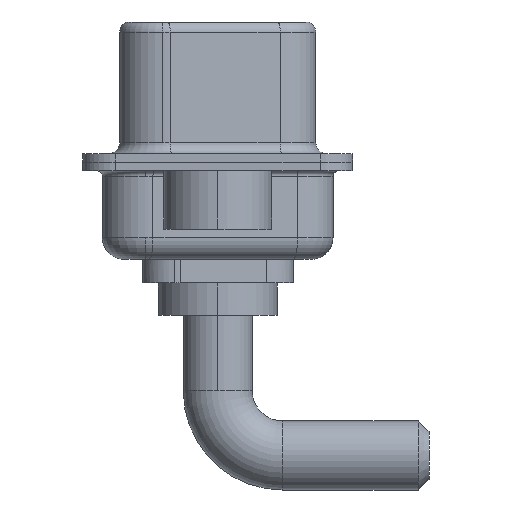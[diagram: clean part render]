
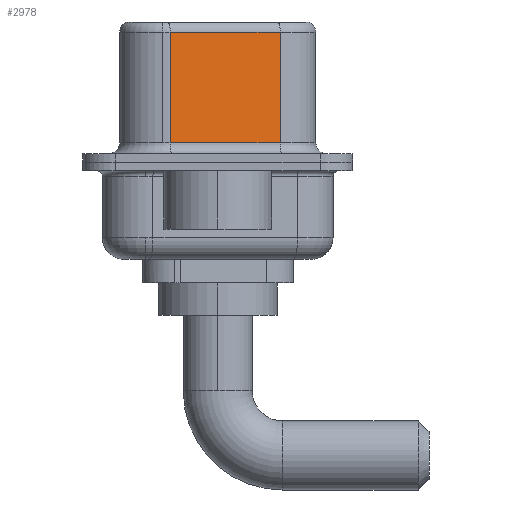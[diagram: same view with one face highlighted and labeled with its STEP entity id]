
A CAD part, left-side view. The second image highlights one B-rep face of the part: STEP entity #2978.
In plain terms, the highlighted planar face has unit normal (-0.985, -0.174, 0).
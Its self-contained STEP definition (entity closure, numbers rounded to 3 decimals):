
#205 = VERTEX_POINT ( 'NONE', #13183 ) ;
#324 = DIRECTION ( 'NONE',  ( 0.174, -0.985, 0. ) ) ;
#850 = ORIENTED_EDGE ( 'NONE', *, *, #14036, .T. ) ;
#1481 = LINE ( 'NONE', #4969, #8563 ) ;
#1835 = ORIENTED_EDGE ( 'NONE', *, *, #7046, .F. ) ;
#1905 = CARTESIAN_POINT ( 'NONE',  ( 4.58, -2.897, 6.52 ) ) ;
#2580 = DIRECTION ( 'NONE',  ( -0.174, 0.985, 0. ) ) ;
#2842 = CARTESIAN_POINT ( 'NONE',  ( 4.58, -2.897, 6.02 ) ) ;
#2854 = LINE ( 'NONE', #1905, #4790 ) ;
#2978 = ADVANCED_FACE ( 'NONE', ( #4484 ), #13265, .F. ) ;
#3888 = VERTEX_POINT ( 'NONE', #6046 ) ;
#3912 = ORIENTED_EDGE ( 'NONE', *, *, #9946, .T. ) ;
#4235 = ORIENTED_EDGE ( 'NONE', *, *, #13758, .T. ) ;
#4484 = FACE_OUTER_BOUND ( 'NONE', #12572, .T. ) ;
#4731 = CARTESIAN_POINT ( 'NONE',  ( 4.58, -2.897, 0.9 ) ) ;
#4790 = VECTOR ( 'NONE', #8615, 1000. ) ;
#4969 = CARTESIAN_POINT ( 'NONE',  ( 4.58, -2.897, 6.02 ) ) ;
#6046 = CARTESIAN_POINT ( 'NONE',  ( 3.68, 2.203, 6.02 ) ) ;
#7046 = EDGE_CURVE ( 'NONE', #9352, #7839, #2854, .T. ) ;
#7706 = DIRECTION ( 'NONE',  ( -0.174, 0.985, 0. ) ) ;
#7839 = VERTEX_POINT ( 'NONE', #4731 ) ;
#8563 = VECTOR ( 'NONE', #2580, 1000. ) ;
#8615 = DIRECTION ( 'NONE',  ( 0., 0., -1. ) ) ;
#8715 = CARTESIAN_POINT ( 'NONE',  ( 3.68, 2.203, 6.52 ) ) ;
#8799 = CARTESIAN_POINT ( 'NONE',  ( 4.58, -2.897, 6.52 ) ) ;
#9156 = CARTESIAN_POINT ( 'NONE',  ( 4.58, -2.897, 0.9 ) ) ;
#9225 = LINE ( 'NONE', #9156, #9562 ) ;
#9352 = VERTEX_POINT ( 'NONE', #2842 ) ;
#9562 = VECTOR ( 'NONE', #324, 1000. ) ;
#9946 = EDGE_CURVE ( 'NONE', #9352, #3888, #1481, .T. ) ;
#10265 = VECTOR ( 'NONE', #13174, 1000. ) ;
#11897 = AXIS2_PLACEMENT_3D ( 'NONE', #8799, #14290, #7706 ) ;
#12157 = LINE ( 'NONE', #8715, #10265 ) ;
#12572 = EDGE_LOOP ( 'NONE', ( #1835, #3912, #850, #4235 ) ) ;
#13174 = DIRECTION ( 'NONE',  ( 0., 0., -1. ) ) ;
#13183 = CARTESIAN_POINT ( 'NONE',  ( 3.68, 2.203, 0.9 ) ) ;
#13265 = PLANE ( 'NONE',  #11897 ) ;
#13758 = EDGE_CURVE ( 'NONE', #205, #7839, #9225, .T. ) ;
#14036 = EDGE_CURVE ( 'NONE', #3888, #205, #12157, .T. ) ;
#14290 = DIRECTION ( 'NONE',  ( 0.985, 0.174, 0. ) ) ;
